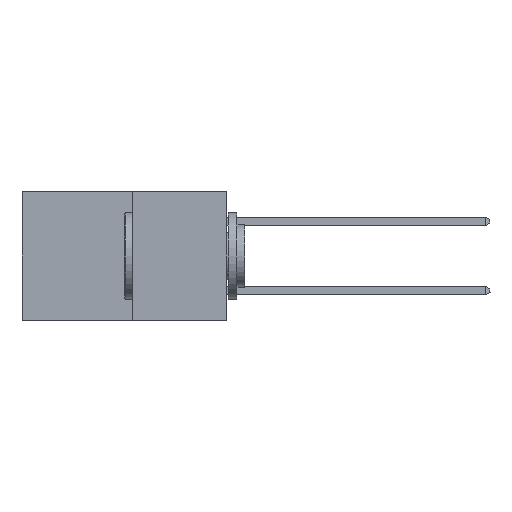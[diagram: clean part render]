
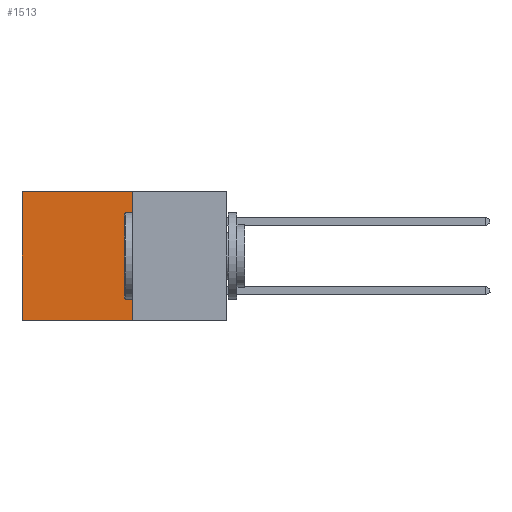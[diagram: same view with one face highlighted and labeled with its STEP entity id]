
A CAD part, left-side view. The second image highlights one B-rep face of the part: STEP entity #1513.
In plain terms, the highlighted planar face has unit normal (-1, 0, 0).
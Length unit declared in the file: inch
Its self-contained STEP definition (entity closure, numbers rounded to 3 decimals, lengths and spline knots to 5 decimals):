
#776 = VERTEX_POINT ( 'NONE', #14337 ) ;
#862 = CARTESIAN_POINT ( 'NONE',  ( 0.277, 0.27, 0. ) ) ;
#925 = VERTEX_POINT ( 'NONE', #862 ) ;
#940 = EDGE_CURVE ( 'NONE', #14803, #776, #14799, .T. ) ;
#1183 = AXIS2_PLACEMENT_3D ( 'NONE', #9842, #6097, #6028 ) ;
#1328 = ORIENTED_EDGE ( 'NONE', *, *, #2872, .F. ) ;
#1362 = DIRECTION ( 'NONE',  ( 0., 1., 0. ) ) ;
#1513 = ADVANCED_FACE ( 'NONE', ( #9353 ), #6159, .F. ) ;
#1659 = CARTESIAN_POINT ( 'NONE',  ( 0.277, 0.27, 0. ) ) ;
#2304 = VECTOR ( 'NONE', #4139, 39.37008 ) ;
#2872 = EDGE_CURVE ( 'NONE', #925, #11076, #5973, .T. ) ;
#4139 = DIRECTION ( 'NONE',  ( 0., 0., -1. ) ) ;
#5499 = ORIENTED_EDGE ( 'NONE', *, *, #7990, .T. ) ;
#5973 = LINE ( 'NONE', #8676, #2304 ) ;
#6028 = DIRECTION ( 'NONE',  ( 0., 0., -1. ) ) ;
#6097 = DIRECTION ( 'NONE',  ( 1., 0., 0. ) ) ;
#6159 = PLANE ( 'NONE',  #1183 ) ;
#6586 = CARTESIAN_POINT ( 'NONE',  ( 0.277, 0.27, -0.37 ) ) ;
#7054 = DIRECTION ( 'NONE',  ( 0., 1., 0. ) ) ;
#7990 = EDGE_CURVE ( 'NONE', #925, #14803, #14601, .T. ) ;
#8676 = CARTESIAN_POINT ( 'NONE',  ( 0.277, 0.27, -0.37 ) ) ;
#8920 = CARTESIAN_POINT ( 'NONE',  ( 0.277, 0.59, 0. ) ) ;
#9353 = FACE_OUTER_BOUND ( 'NONE', #14514, .T. ) ;
#9842 = CARTESIAN_POINT ( 'NONE',  ( 0.277, 0.27, -0.37 ) ) ;
#10649 = DIRECTION ( 'NONE',  ( 0., 0., -1. ) ) ;
#10904 = CARTESIAN_POINT ( 'NONE',  ( 0.277, 0.59, -0.37 ) ) ;
#11076 = VERTEX_POINT ( 'NONE', #6586 ) ;
#11452 = VECTOR ( 'NONE', #7054, 39.37008 ) ;
#12624 = CARTESIAN_POINT ( 'NONE',  ( 0.277, 0.27, -0.37 ) ) ;
#13325 = VECTOR ( 'NONE', #1362, 39.37008 ) ;
#14337 = CARTESIAN_POINT ( 'NONE',  ( 0.277, 0.59, -0.37 ) ) ;
#14380 = VECTOR ( 'NONE', #10649, 39.37008 ) ;
#14514 = EDGE_LOOP ( 'NONE', ( #17296, #17351, #1328, #5499 ) ) ;
#14601 = LINE ( 'NONE', #1659, #13325 ) ;
#14799 = LINE ( 'NONE', #10904, #14380 ) ;
#14803 = VERTEX_POINT ( 'NONE', #8920 ) ;
#15519 = LINE ( 'NONE', #12624, #11452 ) ;
#16292 = EDGE_CURVE ( 'NONE', #11076, #776, #15519, .T. ) ;
#17296 = ORIENTED_EDGE ( 'NONE', *, *, #940, .T. ) ;
#17351 = ORIENTED_EDGE ( 'NONE', *, *, #16292, .F. ) ;
